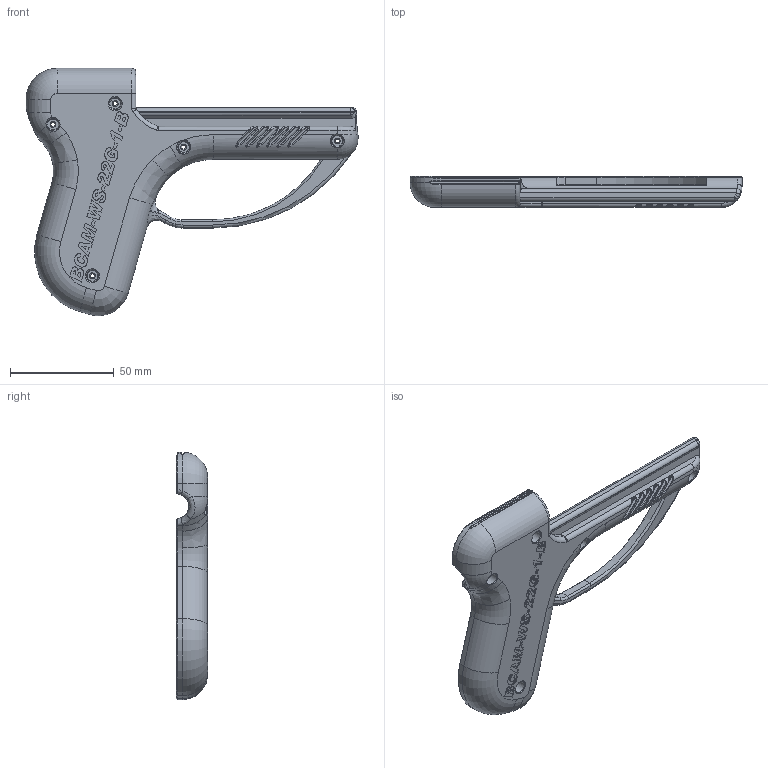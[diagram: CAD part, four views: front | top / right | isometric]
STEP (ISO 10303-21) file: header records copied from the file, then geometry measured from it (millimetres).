
FILE_DESCRIPTION(('FreeCAD Model'),'2;1');
FILE_NAME('Open CASCADE Shape Model','2022-12-07T11:25:01',('Author'),( ''),'Open CASCADE STEP processor 7.6','FreeCAD','Unknown');
FILE_SCHEMA(('AUTOMOTIVE_DESIGN { 1 0 10303 214 1 1 1 1 }'));
Length unit declared in the file: millimetre
Products named in the file (1): Frame-Right
Bounding box: 160 x 15 x 119.19 mm (x, y, z)
Volume: 88839.6 mm3; surface area: 25769.1 mm2
Topology: 1 solids, 1 shells, 573 faces, 1464 edges, 912 vertices
Faces by surface type: plane 214, extrusion 122, bspline 96, cylinder 80, cone 41, torus 16, revolution 4
Full cylindrical faces by diameter (mm): 2 x5, 6 x5
Entity records: 57627 total; most frequent: CARTESIAN_POINT 31691, DIRECTION 3600, ORIENTED_EDGE 2924, PCURVE 2924, DEFINITIONAL_REPRESENTATION 2924, VECTOR 2450, LINE 2328, B_SPLINE_CURVE_WITH_KNOTS 1693
